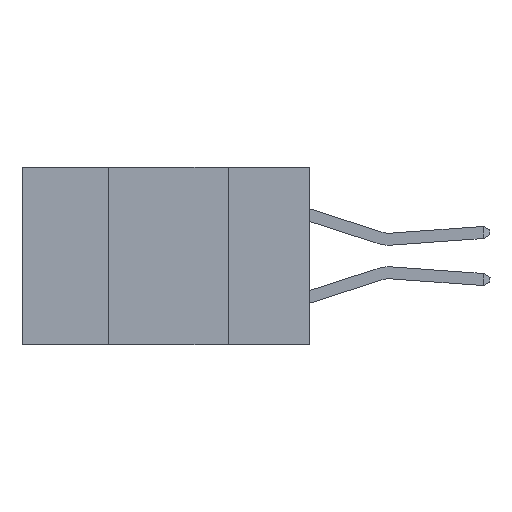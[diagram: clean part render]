
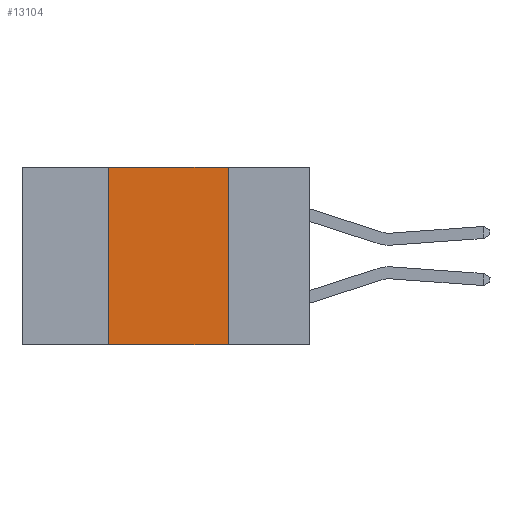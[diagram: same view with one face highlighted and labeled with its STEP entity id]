
A CAD part, left-side view. The second image highlights one B-rep face of the part: STEP entity #13104.
In plain terms, the highlighted planar face has unit normal (-1, 0, 0).
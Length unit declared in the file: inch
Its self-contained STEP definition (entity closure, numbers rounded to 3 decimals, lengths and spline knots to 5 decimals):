
#859 = LINE ( 'NONE', #4481, #13060 ) ;
#2045 = DIRECTION ( 'NONE',  ( 0., -1., 0. ) ) ;
#2077 = CARTESIAN_POINT ( 'NONE',  ( 0., 0.6, 0. ) ) ;
#2782 = VERTEX_POINT ( 'NONE', #15630 ) ;
#4026 = VERTEX_POINT ( 'NONE', #4978 ) ;
#4336 = EDGE_CURVE ( 'NONE', #4026, #16528, #6247, .T. ) ;
#4481 = CARTESIAN_POINT ( 'NONE',  ( 0., 0.17, -0.37 ) ) ;
#4978 = CARTESIAN_POINT ( 'NONE',  ( 0., 0.42, 0. ) ) ;
#6247 = LINE ( 'NONE', #2077, #14370 ) ;
#7003 = PLANE ( 'NONE',  #7490 ) ;
#7317 = FACE_OUTER_BOUND ( 'NONE', #12872, .T. ) ;
#7490 = AXIS2_PLACEMENT_3D ( 'NONE', #9980, #17567, #8515 ) ;
#8485 = VERTEX_POINT ( 'NONE', #14417 ) ;
#8515 = DIRECTION ( 'NONE',  ( 0., 0., -1. ) ) ;
#8934 = CARTESIAN_POINT ( 'NONE',  ( 0., 0.6, -0.37 ) ) ;
#9059 = EDGE_CURVE ( 'NONE', #2782, #4026, #9648, .T. ) ;
#9593 = ORIENTED_EDGE ( 'NONE', *, *, #14906, .F. ) ;
#9648 = LINE ( 'NONE', #17200, #17218 ) ;
#9655 = DIRECTION ( 'NONE',  ( 0., 0., 1. ) ) ;
#9980 = CARTESIAN_POINT ( 'NONE',  ( 0., 0.6, 0. ) ) ;
#10693 = LINE ( 'NONE', #8934, #18235 ) ;
#12071 = DIRECTION ( 'NONE',  ( 0., -1., 0. ) ) ;
#12872 = EDGE_LOOP ( 'NONE', ( #9593, #13595, #17203, #14596 ) ) ;
#13060 = VECTOR ( 'NONE', #15115, 39.37008 ) ;
#13104 = ADVANCED_FACE ( 'NONE', ( #7317 ), #7003, .F. ) ;
#13595 = ORIENTED_EDGE ( 'NONE', *, *, #4336, .F. ) ;
#14370 = VECTOR ( 'NONE', #2045, 39.37008 ) ;
#14417 = CARTESIAN_POINT ( 'NONE',  ( 0., 0.17, -0.37 ) ) ;
#14596 = ORIENTED_EDGE ( 'NONE', *, *, #18634, .T. ) ;
#14906 = EDGE_CURVE ( 'NONE', #16528, #8485, #859, .T. ) ;
#15115 = DIRECTION ( 'NONE',  ( 0., 0., -1. ) ) ;
#15122 = CARTESIAN_POINT ( 'NONE',  ( 0., 0.17, 0. ) ) ;
#15630 = CARTESIAN_POINT ( 'NONE',  ( 0., 0.42, -0.37 ) ) ;
#16528 = VERTEX_POINT ( 'NONE', #15122 ) ;
#17200 = CARTESIAN_POINT ( 'NONE',  ( 0., 0.42, -0.37 ) ) ;
#17203 = ORIENTED_EDGE ( 'NONE', *, *, #9059, .F. ) ;
#17218 = VECTOR ( 'NONE', #9655, 39.37008 ) ;
#17567 = DIRECTION ( 'NONE',  ( 1., 0., 0. ) ) ;
#18235 = VECTOR ( 'NONE', #12071, 39.37008 ) ;
#18634 = EDGE_CURVE ( 'NONE', #2782, #8485, #10693, .T. ) ;
